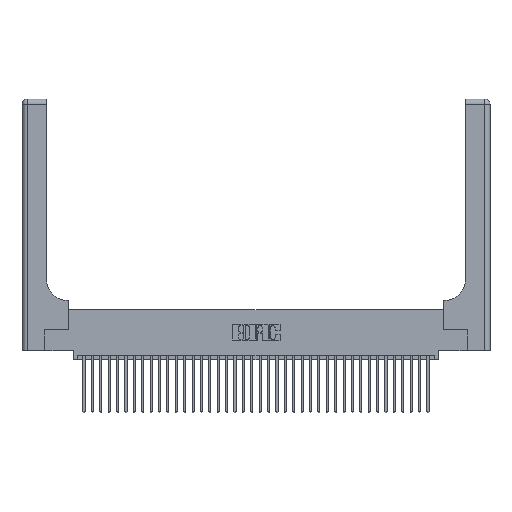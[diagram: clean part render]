
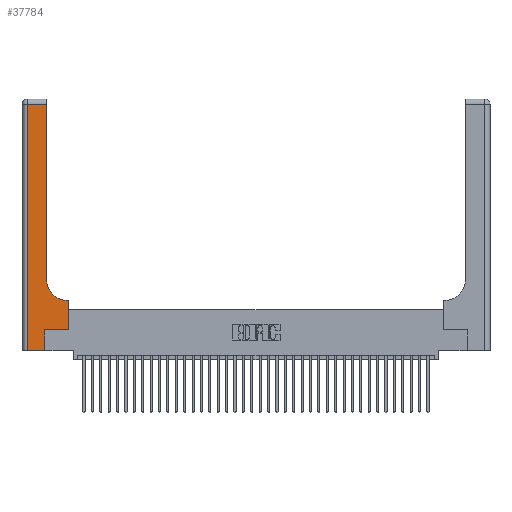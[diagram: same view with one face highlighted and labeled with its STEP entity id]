
A CAD part, top view. The second image highlights one B-rep face of the part: STEP entity #37784.
In plain terms, the highlighted planar face has unit normal (0, 0, 1).
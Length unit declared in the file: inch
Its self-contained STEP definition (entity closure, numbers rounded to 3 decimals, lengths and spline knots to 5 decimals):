
#37 = ORIENTED_EDGE ( 'NONE', *, *, #1017, .T. ) ;
#286 = ORIENTED_EDGE ( 'NONE', *, *, #25892, .T. ) ;
#1017 = EDGE_CURVE ( 'NONE', #15282, #30743, #32185, .T. ) ;
#1769 = VECTOR ( 'NONE', #15369, 39.37008 ) ;
#2078 = ORIENTED_EDGE ( 'NONE', *, *, #11326, .T. ) ;
#2170 = FACE_OUTER_BOUND ( 'NONE', #2414, .T. ) ;
#2414 = EDGE_LOOP ( 'NONE', ( #28742, #26424, #286, #17226, #2078, #35318, #2774, #37, #5395 ) ) ;
#2774 = ORIENTED_EDGE ( 'NONE', *, *, #25222, .T. ) ;
#5364 = LINE ( 'NONE', #34951, #35790 ) ;
#5395 = ORIENTED_EDGE ( 'NONE', *, *, #23923, .T. ) ;
#5548 = DIRECTION ( 'NONE',  ( 0., 1., 0. ) ) ;
#6429 = CARTESIAN_POINT ( 'NONE',  ( 0.2915, 0.85, 0.37 ) ) ;
#6546 = VERTEX_POINT ( 'NONE', #23007 ) ;
#7806 = LINE ( 'NONE', #32364, #30446 ) ;
#8058 = VECTOR ( 'NONE', #19573, 39.37008 ) ;
#8077 = CARTESIAN_POINT ( 'NONE',  ( 0.2915, 2.94, 0.37 ) ) ;
#8320 = VERTEX_POINT ( 'NONE', #35170 ) ;
#8805 = CIRCLE ( 'NONE', #11392, 0.25 ) ;
#9367 = VECTOR ( 'NONE', #36825, 39.37008 ) ;
#9764 = LINE ( 'NONE', #31777, #25459 ) ;
#9842 = PLANE ( 'NONE',  #24756 ) ;
#10085 = CARTESIAN_POINT ( 'NONE',  ( 0.269, 0.25, 0.37 ) ) ;
#10341 = VERTEX_POINT ( 'NONE', #23665 ) ;
#10711 = CARTESIAN_POINT ( 'NONE',  ( 0.06, 2.94, 0.37 ) ) ;
#11326 = EDGE_CURVE ( 'NONE', #6546, #20556, #9764, .T. ) ;
#11392 = AXIS2_PLACEMENT_3D ( 'NONE', #14960, #35471, #17940 ) ;
#12815 = DIRECTION ( 'NONE',  ( 0., 0., -1. ) ) ;
#14172 = DIRECTION ( 'NONE',  ( 0., 1., 0. ) ) ;
#14960 = CARTESIAN_POINT ( 'NONE',  ( 0.5415, 0.85, 0.37 ) ) ;
#15282 = VERTEX_POINT ( 'NONE', #26586 ) ;
#15369 = DIRECTION ( 'NONE',  ( 0., -1., 0. ) ) ;
#15607 = EDGE_CURVE ( 'NONE', #20556, #10341, #23260, .T. ) ;
#16616 = CARTESIAN_POINT ( 'NONE',  ( 0., 0., 0.37 ) ) ;
#17226 = ORIENTED_EDGE ( 'NONE', *, *, #21651, .T. ) ;
#17855 = CARTESIAN_POINT ( 'NONE',  ( 0.5585, 0.25, 0.37 ) ) ;
#17940 = DIRECTION ( 'NONE',  ( 1., 0., 0. ) ) ;
#19573 = DIRECTION ( 'NONE',  ( 1., 0., 0. ) ) ;
#20556 = VERTEX_POINT ( 'NONE', #35251 ) ;
#21651 = EDGE_CURVE ( 'NONE', #8320, #6546, #32516, .T. ) ;
#22335 = VECTOR ( 'NONE', #33642, 39.37008 ) ;
#23007 = CARTESIAN_POINT ( 'NONE',  ( 0.269, 0., 0.37 ) ) ;
#23260 = LINE ( 'NONE', #10085, #22335 ) ;
#23612 = VERTEX_POINT ( 'NONE', #10711 ) ;
#23665 = CARTESIAN_POINT ( 'NONE',  ( 0.5585, 0.25, 0.37 ) ) ;
#23923 = EDGE_CURVE ( 'NONE', #30743, #29042, #8805, .T. ) ;
#24377 = VECTOR ( 'NONE', #33431, 39.37008 ) ;
#24756 = AXIS2_PLACEMENT_3D ( 'NONE', #36183, #12815, #33401 ) ;
#25222 = EDGE_CURVE ( 'NONE', #10341, #15282, #32875, .T. ) ;
#25459 = VECTOR ( 'NONE', #14172, 39.37008 ) ;
#25480 = LINE ( 'NONE', #30011, #1769 ) ;
#25892 = EDGE_CURVE ( 'NONE', #23612, #8320, #25480, .T. ) ;
#26424 = ORIENTED_EDGE ( 'NONE', *, *, #35679, .T. ) ;
#26586 = CARTESIAN_POINT ( 'NONE',  ( 0.5585, 0.6, 0.37 ) ) ;
#27502 = VERTEX_POINT ( 'NONE', #8077 ) ;
#28306 = EDGE_CURVE ( 'NONE', #29042, #27502, #5364, .T. ) ;
#28742 = ORIENTED_EDGE ( 'NONE', *, *, #28306, .T. ) ;
#29042 = VERTEX_POINT ( 'NONE', #6429 ) ;
#30011 = CARTESIAN_POINT ( 'NONE',  ( 0.06, 3., 0.37 ) ) ;
#30446 = VECTOR ( 'NONE', #35282, 39.37008 ) ;
#30474 = CARTESIAN_POINT ( 'NONE',  ( 0.2915, 0.6, 0.37 ) ) ;
#30743 = VERTEX_POINT ( 'NONE', #32643 ) ;
#31777 = CARTESIAN_POINT ( 'NONE',  ( 0.269, 0., 0.37 ) ) ;
#32185 = LINE ( 'NONE', #30474, #24377 ) ;
#32364 = CARTESIAN_POINT ( 'NONE',  ( 0., 2.94, 0.37 ) ) ;
#32516 = LINE ( 'NONE', #16616, #8058 ) ;
#32643 = CARTESIAN_POINT ( 'NONE',  ( 0.5415, 0.6, 0.37 ) ) ;
#32875 = LINE ( 'NONE', #17855, #9367 ) ;
#33401 = DIRECTION ( 'NONE',  ( -1., 0., 0. ) ) ;
#33431 = DIRECTION ( 'NONE',  ( -1., 0., 0. ) ) ;
#33642 = DIRECTION ( 'NONE',  ( 1., 0., 0. ) ) ;
#34951 = CARTESIAN_POINT ( 'NONE',  ( 0.2915, 3., 0.37 ) ) ;
#35170 = CARTESIAN_POINT ( 'NONE',  ( 0.06, 0., 0.37 ) ) ;
#35251 = CARTESIAN_POINT ( 'NONE',  ( 0.269, 0.25, 0.37 ) ) ;
#35282 = DIRECTION ( 'NONE',  ( -1., 0., 0. ) ) ;
#35318 = ORIENTED_EDGE ( 'NONE', *, *, #15607, .T. ) ;
#35471 = DIRECTION ( 'NONE',  ( 0., 0., -1. ) ) ;
#35679 = EDGE_CURVE ( 'NONE', #27502, #23612, #7806, .T. ) ;
#35790 = VECTOR ( 'NONE', #5548, 39.37008 ) ;
#36183 = CARTESIAN_POINT ( 'NONE',  ( 0., 3., 0.37 ) ) ;
#36825 = DIRECTION ( 'NONE',  ( 0., 1., 0. ) ) ;
#37784 = ADVANCED_FACE ( 'NONE', ( #2170 ), #9842, .F. ) ;
